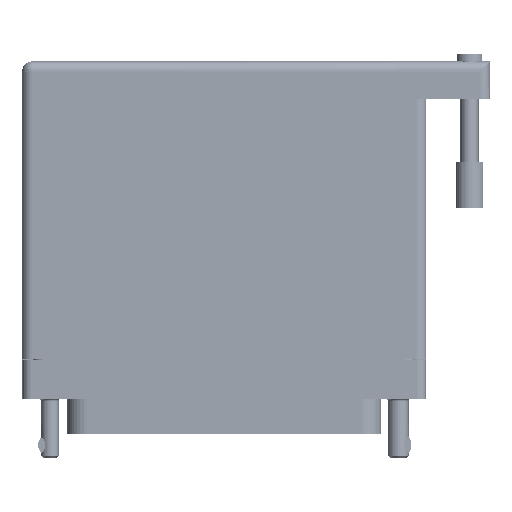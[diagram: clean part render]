
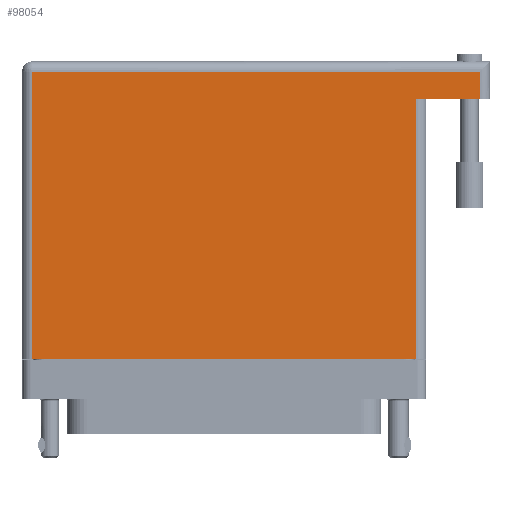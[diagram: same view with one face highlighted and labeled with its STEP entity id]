
A CAD part, front view. The second image highlights one B-rep face of the part: STEP entity #98054.
In plain terms, the highlighted face is planar.
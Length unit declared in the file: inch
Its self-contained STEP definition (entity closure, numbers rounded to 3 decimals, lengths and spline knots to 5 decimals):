
#3257 = ORIENTED_EDGE ( 'NONE', *, *, #62174, .T. ) ;
#3321 = VECTOR ( 'NONE', #4821, 39.37008 ) ;
#4519 = CARTESIAN_POINT ( 'NONE',  ( -1.3775, 1.93, 0.765 ) ) ;
#4821 = DIRECTION ( 'NONE',  ( 1., 0., 0. ) ) ;
#5115 = CARTESIAN_POINT ( 'NONE',  ( -1.3775, 1.86, 0.765 ) ) ;
#5872 = VECTOR ( 'NONE', #27773, 39.37008 ) ;
#6740 = LINE ( 'NONE', #5115, #57632 ) ;
#10717 = LINE ( 'NONE', #51969, #18055 ) ;
#16550 = VERTEX_POINT ( 'NONE', #46198 ) ;
#18055 = VECTOR ( 'NONE', #74929, 39.37008 ) ;
#26850 = VECTOR ( 'NONE', #55390, 39.37008 ) ;
#27773 = DIRECTION ( 'NONE',  ( -1., 0., 0. ) ) ;
#28266 = CARTESIAN_POINT ( 'NONE',  ( -1.3075, -0.1, 0.765 ) ) ;
#30762 = EDGE_CURVE ( 'NONE', #55299, #16550, #6740, .T. ) ;
#31077 = VERTEX_POINT ( 'NONE', #68288 ) ;
#39855 = EDGE_CURVE ( 'NONE', #66453, #100155, #59316, .T. ) ;
#39999 = EDGE_CURVE ( 'NONE', #94293, #31077, #51850, .T. ) ;
#44883 = PLANE ( 'NONE',  #75163 ) ;
#46198 = CARTESIAN_POINT ( 'NONE',  ( -1.3075, 1.86, 0.765 ) ) ;
#46304 = ORIENTED_EDGE ( 'NONE', *, *, #30762, .T. ) ;
#51418 = EDGE_LOOP ( 'NONE', ( #84744, #60431, #75036, #93468, #46304, #3257 ) ) ;
#51619 = EDGE_CURVE ( 'NONE', #66453, #55299, #10717, .T. ) ;
#51850 = LINE ( 'NONE', #61464, #3321 ) ;
#51969 = CARTESIAN_POINT ( 'NONE',  ( 1.7425, 1.93, 0.765 ) ) ;
#55299 = VERTEX_POINT ( 'NONE', #89000 ) ;
#55390 = DIRECTION ( 'NONE',  ( 0., 1., 0. ) ) ;
#57632 = VECTOR ( 'NONE', #92335, 39.37008 ) ;
#59316 = LINE ( 'NONE', #91360, #5872 ) ;
#60431 = ORIENTED_EDGE ( 'NONE', *, *, #79789, .T. ) ;
#60673 = FACE_OUTER_BOUND ( 'NONE', #51418, .T. ) ;
#61464 = CARTESIAN_POINT ( 'NONE',  ( -1.3775, -0.1, 0.765 ) ) ;
#62174 = EDGE_CURVE ( 'NONE', #16550, #94293, #78585, .T. ) ;
#64108 = LINE ( 'NONE', #80422, #26850 ) ;
#66453 = VERTEX_POINT ( 'NONE', #102688 ) ;
#68288 = CARTESIAN_POINT ( 'NONE',  ( 1.3075, -0.1, 0.765 ) ) ;
#74929 = DIRECTION ( 'NONE',  ( 0., 1., 0. ) ) ;
#75036 = ORIENTED_EDGE ( 'NONE', *, *, #39855, .F. ) ;
#75163 = AXIS2_PLACEMENT_3D ( 'NONE', #4519, #83487, #84165 ) ;
#75797 = CARTESIAN_POINT ( 'NONE',  ( -1.3075, -0.1, 0.765 ) ) ;
#78585 = LINE ( 'NONE', #28266, #92181 ) ;
#79789 = EDGE_CURVE ( 'NONE', #31077, #100155, #64108, .T. ) ;
#80422 = CARTESIAN_POINT ( 'NONE',  ( 1.3075, 1.674, 0.765 ) ) ;
#83487 = DIRECTION ( 'NONE',  ( 0., 0., -1. ) ) ;
#83896 = DIRECTION ( 'NONE',  ( 0., -1., 0. ) ) ;
#84165 = DIRECTION ( 'NONE',  ( -1., 0., 0. ) ) ;
#84744 = ORIENTED_EDGE ( 'NONE', *, *, #39999, .T. ) ;
#89000 = CARTESIAN_POINT ( 'NONE',  ( 1.7425, 1.86, 0.765 ) ) ;
#91360 = CARTESIAN_POINT ( 'NONE',  ( 1.8125, 1.674, 0.765 ) ) ;
#92181 = VECTOR ( 'NONE', #83896, 39.37008 ) ;
#92335 = DIRECTION ( 'NONE',  ( -1., 0., 0. ) ) ;
#93468 = ORIENTED_EDGE ( 'NONE', *, *, #51619, .T. ) ;
#94293 = VERTEX_POINT ( 'NONE', #75797 ) ;
#95653 = CARTESIAN_POINT ( 'NONE',  ( 1.3075, 1.674, 0.765 ) ) ;
#98054 = ADVANCED_FACE ( 'NONE', ( #60673 ), #44883, .F. ) ;
#100155 = VERTEX_POINT ( 'NONE', #95653 ) ;
#102688 = CARTESIAN_POINT ( 'NONE',  ( 1.7425, 1.674, 0.765 ) ) ;
